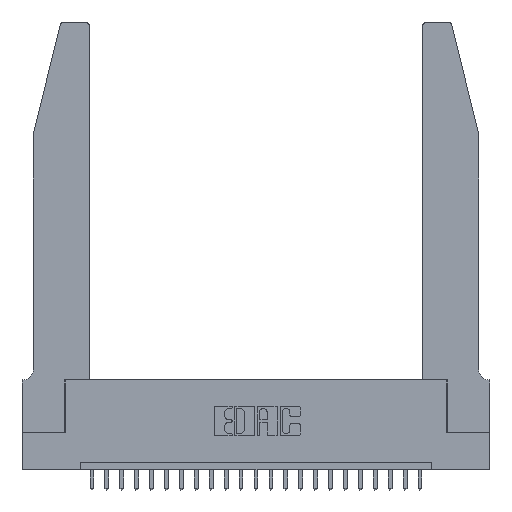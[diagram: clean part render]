
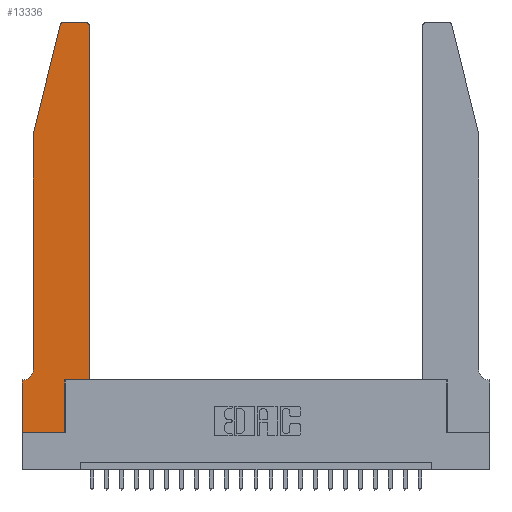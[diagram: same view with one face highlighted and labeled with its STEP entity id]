
A CAD part, top view. The second image highlights one B-rep face of the part: STEP entity #13336.
In plain terms, the highlighted planar face has unit normal (0, 0, 1).
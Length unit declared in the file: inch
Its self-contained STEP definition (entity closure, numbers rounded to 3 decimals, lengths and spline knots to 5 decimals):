
#222 = VERTEX_POINT ( 'NONE', #22986 ) ;
#744 = LINE ( 'NONE', #5350, #4312 ) ;
#857 = VECTOR ( 'NONE', #3127, 39.37008 ) ;
#1174 = EDGE_LOOP ( 'NONE', ( #9589, #22455, #22338, #15032, #23074, #8977, #3494, #2389, #8231, #4265, #7594, #17973 ) ) ;
#1641 = DIRECTION ( 'NONE',  ( 1., 0., 0. ) ) ;
#1687 = EDGE_CURVE ( 'NONE', #16261, #14604, #17645, .T. ) ;
#1810 = LINE ( 'NONE', #14951, #19063 ) ;
#2389 = ORIENTED_EDGE ( 'NONE', *, *, #18723, .T. ) ;
#2600 = LINE ( 'NONE', #20156, #9076 ) ;
#2627 = CARTESIAN_POINT ( 'NONE',  ( 0.0755, 2., 0.37 ) ) ;
#2655 = VERTEX_POINT ( 'NONE', #24452 ) ;
#2683 = DIRECTION ( 'NONE',  ( 0., 0., 1. ) ) ;
#3041 = VECTOR ( 'NONE', #19144, 39.37008 ) ;
#3127 = DIRECTION ( 'NONE',  ( 1., 0., 0. ) ) ;
#3486 = CARTESIAN_POINT ( 'NONE',  ( 0.2605, 2.75, 0.37 ) ) ;
#3494 = ORIENTED_EDGE ( 'NONE', *, *, #8020, .T. ) ;
#3522 = EDGE_CURVE ( 'NONE', #2655, #16030, #1810, .T. ) ;
#3716 = DIRECTION ( 'NONE',  ( -1., 0., 0. ) ) ;
#3740 = EDGE_CURVE ( 'NONE', #21584, #21222, #5930, .T. ) ;
#3883 = CARTESIAN_POINT ( 'NONE',  ( 0.0755, 0.42, 0.37 ) ) ;
#4265 = ORIENTED_EDGE ( 'NONE', *, *, #3522, .T. ) ;
#4312 = VECTOR ( 'NONE', #5276, 39.37008 ) ;
#5057 = CARTESIAN_POINT ( 'NONE',  ( 0.4505, 2.72, 0.37 ) ) ;
#5276 = DIRECTION ( 'NONE',  ( 0., 1., 0. ) ) ;
#5350 = CARTESIAN_POINT ( 'NONE',  ( 0.4505, 0.35, 0.37 ) ) ;
#5685 = VERTEX_POINT ( 'NONE', #3883 ) ;
#5799 = AXIS2_PLACEMENT_3D ( 'NONE', #13751, #2683, #10113 ) ;
#5930 = CIRCLE ( 'NONE', #24531, 0.03 ) ;
#6286 = DIRECTION ( 'NONE',  ( 0., 0., 1. ) ) ;
#6364 = EDGE_CURVE ( 'NONE', #14604, #21584, #18951, .T. ) ;
#6613 = EDGE_CURVE ( 'NONE', #22657, #5685, #2600, .T. ) ;
#6878 = VECTOR ( 'NONE', #10302, 39.37008 ) ;
#7128 = CARTESIAN_POINT ( 'NONE',  ( 0., 0., 0.37 ) ) ;
#7343 = VERTEX_POINT ( 'NONE', #16550 ) ;
#7594 = ORIENTED_EDGE ( 'NONE', *, *, #21181, .T. ) ;
#7921 = CARTESIAN_POINT ( 'NONE',  ( 0.4505, 0.35, 0.37 ) ) ;
#8020 = EDGE_CURVE ( 'NONE', #222, #7343, #20661, .T. ) ;
#8204 = PLANE ( 'NONE',  #5799 ) ;
#8231 = ORIENTED_EDGE ( 'NONE', *, *, #16161, .T. ) ;
#8296 = AXIS2_PLACEMENT_3D ( 'NONE', #18585, #13428, #15349 ) ;
#8977 = ORIENTED_EDGE ( 'NONE', *, *, #16866, .T. ) ;
#9060 = CARTESIAN_POINT ( 'NONE',  ( 0.25487, 2.72718, 0.37 ) ) ;
#9076 = VECTOR ( 'NONE', #24070, 39.37008 ) ;
#9589 = ORIENTED_EDGE ( 'NONE', *, *, #6364, .T. ) ;
#10113 = DIRECTION ( 'NONE',  ( 1., 0., 0. ) ) ;
#10244 = EDGE_CURVE ( 'NONE', #5685, #23742, #22941, .T. ) ;
#10302 = DIRECTION ( 'NONE',  ( -0.239, -0.971, 0. ) ) ;
#10592 = CARTESIAN_POINT ( 'NONE',  ( 0.2865, 0.35, 0.37 ) ) ;
#11298 = LINE ( 'NONE', #15250, #3041 ) ;
#11923 = DIRECTION ( 'NONE',  ( 1., 0., 0. ) ) ;
#12009 = CARTESIAN_POINT ( 'NONE',  ( 0.284, 2.72, 0.37 ) ) ;
#12557 = VECTOR ( 'NONE', #14947, 39.37008 ) ;
#13336 = ADVANCED_FACE ( 'NONE', ( #18917 ), #8204, .T. ) ;
#13428 = DIRECTION ( 'NONE',  ( 0., 0., -1. ) ) ;
#13751 = CARTESIAN_POINT ( 'NONE',  ( 0., 0.35, 0.37 ) ) ;
#14072 = AXIS2_PLACEMENT_3D ( 'NONE', #17465, #15586, #15336 ) ;
#14102 = CARTESIAN_POINT ( 'NONE',  ( 0.4205, 2.75, 0.37 ) ) ;
#14414 = CARTESIAN_POINT ( 'NONE',  ( 0.2865, 0., 0.37 ) ) ;
#14604 = VERTEX_POINT ( 'NONE', #14102 ) ;
#14947 = DIRECTION ( 'NONE',  ( 0., -1., 0. ) ) ;
#14951 = CARTESIAN_POINT ( 'NONE',  ( 0.4505, 0.35, 0.37 ) ) ;
#15032 = ORIENTED_EDGE ( 'NONE', *, *, #6613, .T. ) ;
#15250 = CARTESIAN_POINT ( 'NONE',  ( 0.0755, 0.35, 0.37 ) ) ;
#15336 = DIRECTION ( 'NONE',  ( 1., 0., 0. ) ) ;
#15349 = DIRECTION ( 'NONE',  ( -1., 0., 0. ) ) ;
#15586 = DIRECTION ( 'NONE',  ( 0., 0., 1. ) ) ;
#16030 = VERTEX_POINT ( 'NONE', #7921 ) ;
#16161 = EDGE_CURVE ( 'NONE', #17642, #2655, #24487, .T. ) ;
#16261 = VERTEX_POINT ( 'NONE', #5057 ) ;
#16550 = CARTESIAN_POINT ( 'NONE',  ( 0., 0., 0.37 ) ) ;
#16646 = EDGE_CURVE ( 'NONE', #21222, #22657, #21486, .T. ) ;
#16866 = EDGE_CURVE ( 'NONE', #23742, #222, #11298, .T. ) ;
#17154 = VECTOR ( 'NONE', #3716, 39.37008 ) ;
#17465 = CARTESIAN_POINT ( 'NONE',  ( 0.4205, 2.72, 0.37 ) ) ;
#17642 = VERTEX_POINT ( 'NONE', #14414 ) ;
#17645 = CIRCLE ( 'NONE', #14072, 0.03 ) ;
#17973 = ORIENTED_EDGE ( 'NONE', *, *, #1687, .T. ) ;
#18532 = VECTOR ( 'NONE', #23956, 39.37008 ) ;
#18585 = CARTESIAN_POINT ( 'NONE',  ( 0.0055, 0.42, 0.37 ) ) ;
#18638 = CARTESIAN_POINT ( 'NONE',  ( 0.0755, 2., 0.37 ) ) ;
#18723 = EDGE_CURVE ( 'NONE', #7343, #17642, #24057, .T. ) ;
#18917 = FACE_OUTER_BOUND ( 'NONE', #1174, .T. ) ;
#18951 = LINE ( 'NONE', #3486, #17154 ) ;
#19063 = VECTOR ( 'NONE', #1641, 39.37008 ) ;
#19144 = DIRECTION ( 'NONE',  ( -1., 0., 0. ) ) ;
#19768 = CARTESIAN_POINT ( 'NONE',  ( 0.0055, 0.35, 0.37 ) ) ;
#20156 = CARTESIAN_POINT ( 'NONE',  ( 0.0755, 2., 0.37 ) ) ;
#20661 = LINE ( 'NONE', #22428, #12557 ) ;
#21181 = EDGE_CURVE ( 'NONE', #16030, #16261, #744, .T. ) ;
#21222 = VERTEX_POINT ( 'NONE', #9060 ) ;
#21325 = CARTESIAN_POINT ( 'NONE',  ( 0.284, 2.75, 0.37 ) ) ;
#21486 = LINE ( 'NONE', #2627, #6878 ) ;
#21584 = VERTEX_POINT ( 'NONE', #21325 ) ;
#22338 = ORIENTED_EDGE ( 'NONE', *, *, #16646, .T. ) ;
#22428 = CARTESIAN_POINT ( 'NONE',  ( 0., 0., 0.37 ) ) ;
#22455 = ORIENTED_EDGE ( 'NONE', *, *, #3740, .T. ) ;
#22657 = VERTEX_POINT ( 'NONE', #18638 ) ;
#22941 = CIRCLE ( 'NONE', #8296, 0.07 ) ;
#22986 = CARTESIAN_POINT ( 'NONE',  ( 0., 0.35, 0.37 ) ) ;
#23074 = ORIENTED_EDGE ( 'NONE', *, *, #10244, .T. ) ;
#23742 = VERTEX_POINT ( 'NONE', #19768 ) ;
#23956 = DIRECTION ( 'NONE',  ( 0., 1., 0. ) ) ;
#24057 = LINE ( 'NONE', #7128, #857 ) ;
#24070 = DIRECTION ( 'NONE',  ( 0., -1., 0. ) ) ;
#24452 = CARTESIAN_POINT ( 'NONE',  ( 0.2865, 0.35, 0.37 ) ) ;
#24487 = LINE ( 'NONE', #10592, #18532 ) ;
#24531 = AXIS2_PLACEMENT_3D ( 'NONE', #12009, #6286, #11923 ) ;
